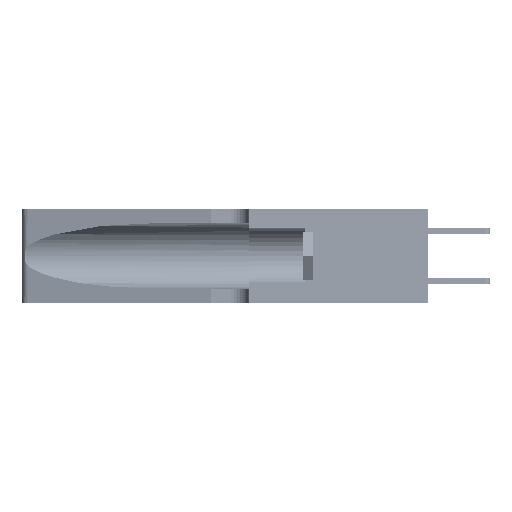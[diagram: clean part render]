
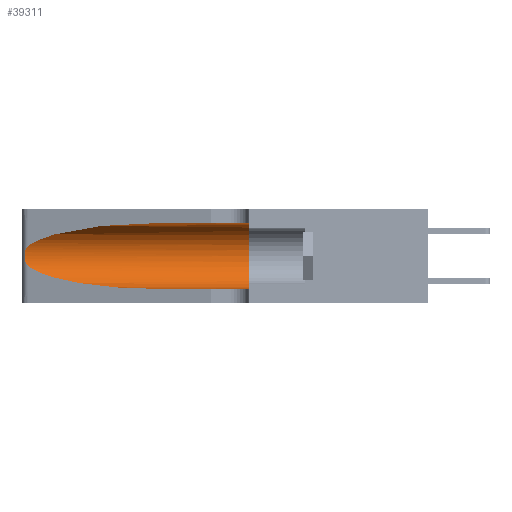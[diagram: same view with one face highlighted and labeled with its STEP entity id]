
A CAD part, left-side view. The second image highlights one B-rep face of the part: STEP entity #39311.
In plain terms, the highlighted cylindrical face has radius 3.308 mm (diameter 6.617 mm), a partial arc.
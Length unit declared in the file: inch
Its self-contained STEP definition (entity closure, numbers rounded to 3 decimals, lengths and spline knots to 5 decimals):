
#856 = CARTESIAN_POINT ( 'NONE',  ( 0.25487, 1.22718, 0.14631 ) ) ;
#864 = CARTESIAN_POINT ( 'NONE',  ( 0.26018, 1.23835, 0.19895 ) ) ;
#1030 = CARTESIAN_POINT ( 'NONE',  ( 0.25639, 1.23186, 0.15144 ) ) ;
#3380 = EDGE_CURVE ( 'NONE', #33077, #28652, #33809, .T. ) ;
#4435 = CARTESIAN_POINT ( 'NONE',  ( 0.25487, 1.22718, 0.22369 ) ) ;
#5006 = CARTESIAN_POINT ( 'NONE',  ( 0.1305, 0.72297, 0.31525 ) ) ;
#7032 = LINE ( 'NONE', #33057, #11878 ) ;
#9115 = VERTEX_POINT ( 'NONE', #37244 ) ;
#11878 = VECTOR ( 'NONE', #26705, 39.37008 ) ;
#13365 = DIRECTION ( 'NONE',  ( 0., 0., -1. ) ) ;
#13494 = VECTOR ( 'NONE', #28156, 39.37008 ) ;
#14922 = CARTESIAN_POINT ( 'NONE',  ( 0.25487, 1.22718, 0.22369 ) ) ;
#15297 = CARTESIAN_POINT ( 'NONE',  ( 0.18966, 0.96281, 0.31525 ) ) ;
#16400 = AXIS2_PLACEMENT_3D ( 'NONE', #27247, #41027, #13365 ) ;
#16528 = EDGE_CURVE ( 'NONE', #16928, #9115, #38732, .T. ) ;
#16928 = VERTEX_POINT ( 'NONE', #14922 ) ;
#17335 = VERTEX_POINT ( 'NONE', #18814 ) ;
#17769 = CYLINDRICAL_SURFACE ( 'NONE', #16400, 0.13025 ) ;
#18388 = CARTESIAN_POINT ( 'NONE',  ( 0.26075, 1.23896, 0.178 ) ) ;
#18554 = CARTESIAN_POINT ( 'NONE',  ( 0.26017, 1.23833, 0.17102 ) ) ;
#18814 = CARTESIAN_POINT ( 'NONE',  ( 0.1305, 0.72297, 0.05475 ) ) ;
#18815 = CARTESIAN_POINT ( 'NONE',  ( 0.25487, 1.22718, 0.22369 ) ) ;
#18960 = AXIS2_PLACEMENT_3D ( 'NONE', #43205, #30628, #28528 ) ;
#19768 = CARTESIAN_POINT ( 'NONE',  ( 0.2373, 1.15595, 0.28018 ) ) ;
#20797 = EDGE_LOOP ( 'NONE', ( #33346, #26966, #39984, #40620, #31125, #29837 ) ) ;
#23490 = EDGE_CURVE ( 'NONE', #33982, #16928, #32077, .T. ) ;
#25206 = CARTESIAN_POINT ( 'NONE',  ( 0.18966, 0.96281, 0.05475 ) ) ;
#25362 = CARTESIAN_POINT ( 'NONE',  ( 0.25854, 1.2359, 0.20912 ) ) ;
#26572 = LINE ( 'NONE', #38597, #13494 ) ;
#26705 = DIRECTION ( 'NONE',  ( 0., -1., 0. ) ) ;
#26966 = ORIENTED_EDGE ( 'NONE', *, *, #16528, .T. ) ;
#27247 = CARTESIAN_POINT ( 'NONE',  ( 0.1305, 1.61858, 0.185 ) ) ;
#28156 = DIRECTION ( 'NONE',  ( 0., -1., 0. ) ) ;
#28285 = CARTESIAN_POINT ( 'NONE',  ( 0.2373, 1.15595, 0.08982 ) ) ;
#28352 = CARTESIAN_POINT ( 'NONE',  ( 0.1305, 0.35, 0.05475 ) ) ;
#28528 = DIRECTION ( 'NONE',  ( 0., 0., 1. ) ) ;
#28588 = CARTESIAN_POINT ( 'NONE',  ( 0.25555, 1.22994, 0.2215 ) ) ;
#28652 = VERTEX_POINT ( 'NONE', #28352 ) ;
#28748 = CARTESIAN_POINT ( 'NONE',  ( 0.26075, 1.23896, 0.19203 ) ) ;
#29837 = ORIENTED_EDGE ( 'NONE', *, *, #38355, .F. ) ;
#30628 = DIRECTION ( 'NONE',  ( 0., 1., 0. ) ) ;
#31125 = ORIENTED_EDGE ( 'NONE', *, *, #3380, .F. ) ;
#32077 =( BOUNDED_CURVE ( )  B_SPLINE_CURVE ( 3, ( #32080, #15297, #19768, #18815 ),
 .UNSPECIFIED., .F., .T. ) 
 B_SPLINE_CURVE_WITH_KNOTS ( ( 4, 4 ),
 ( 1.5708, 2.84003 ),
 .UNSPECIFIED. ) 
 CURVE ( )  GEOMETRIC_REPRESENTATION_ITEM ( )  RATIONAL_B_SPLINE_CURVE ( ( 1., 0.87, 0.87, 1. ) ) 
 REPRESENTATION_ITEM ( '' )  );
#32080 = CARTESIAN_POINT ( 'NONE',  ( 0.1305, 0.72297, 0.31525 ) ) ;
#32223 = CARTESIAN_POINT ( 'NONE',  ( 0.25856, 1.23593, 0.16098 ) ) ;
#33057 = CARTESIAN_POINT ( 'NONE',  ( 0.1305, 1.61858, 0.31525 ) ) ;
#33077 = VERTEX_POINT ( 'NONE', #34760 ) ;
#33346 = ORIENTED_EDGE ( 'NONE', *, *, #23490, .T. ) ;
#33809 = CIRCLE ( 'NONE', #18960, 0.13025 ) ;
#33982 = VERTEX_POINT ( 'NONE', #5006 ) ;
#34760 = CARTESIAN_POINT ( 'NONE',  ( 0.1305, 0.35, 0.31525 ) ) ;
#35385 =( BOUNDED_CURVE ( )  B_SPLINE_CURVE ( 3, ( #856, #28285, #25206, #42080 ),
 .UNSPECIFIED., .F., .F. ) 
 B_SPLINE_CURVE_WITH_KNOTS ( ( 4, 4 ),
 ( 3.44316, 4.71239 ),
 .UNSPECIFIED. ) 
 CURVE ( )  GEOMETRIC_REPRESENTATION_ITEM ( )  RATIONAL_B_SPLINE_CURVE ( ( 1., 0.87, 0.87, 1. ) ) 
 REPRESENTATION_ITEM ( '' )  );
#35833 = CARTESIAN_POINT ( 'NONE',  ( 0.25787, 1.23484, 0.2124 ) ) ;
#37041 = EDGE_CURVE ( 'NONE', #9115, #17335, #35385, .T. ) ;
#37244 = CARTESIAN_POINT ( 'NONE',  ( 0.25487, 1.22718, 0.14631 ) ) ;
#38355 = EDGE_CURVE ( 'NONE', #33982, #33077, #7032, .T. ) ;
#38597 = CARTESIAN_POINT ( 'NONE',  ( 0.1305, 1.61858, 0.05475 ) ) ;
#38644 = EDGE_CURVE ( 'NONE', #17335, #28652, #26572, .T. ) ;
#38732 = B_SPLINE_CURVE_WITH_KNOTS ( 'NONE', 3,
 ( #4435, #28588, #39199, #35833, #25362, #864, #28748, #18388, #18554, #32223, #42683, #1030, #42996, #42831 ),
 .UNSPECIFIED., .F., .F.,
 ( 4, 2, 2, 2, 2, 2, 4 ),
 ( 0., 0.00027, 0.00053, 0.00107, 0.0016, 0.00187, 0.00214 ),
 .UNSPECIFIED. ) ;
#39199 = CARTESIAN_POINT ( 'NONE',  ( 0.25639, 1.23184, 0.21858 ) ) ;
#39311 = ADVANCED_FACE ( 'NONE', ( #41745 ), #17769, .F. ) ;
#39984 = ORIENTED_EDGE ( 'NONE', *, *, #37041, .T. ) ;
#40620 = ORIENTED_EDGE ( 'NONE', *, *, #38644, .T. ) ;
#41027 = DIRECTION ( 'NONE',  ( 0., -1., 0. ) ) ;
#41745 = FACE_OUTER_BOUND ( 'NONE', #20797, .T. ) ;
#42080 = CARTESIAN_POINT ( 'NONE',  ( 0.1305, 0.72297, 0.05475 ) ) ;
#42683 = CARTESIAN_POINT ( 'NONE',  ( 0.25789, 1.23486, 0.15765 ) ) ;
#42831 = CARTESIAN_POINT ( 'NONE',  ( 0.25487, 1.22718, 0.14631 ) ) ;
#42996 = CARTESIAN_POINT ( 'NONE',  ( 0.25555, 1.22993, 0.14849 ) ) ;
#43205 = CARTESIAN_POINT ( 'NONE',  ( 0.1305, 0.35, 0.185 ) ) ;
